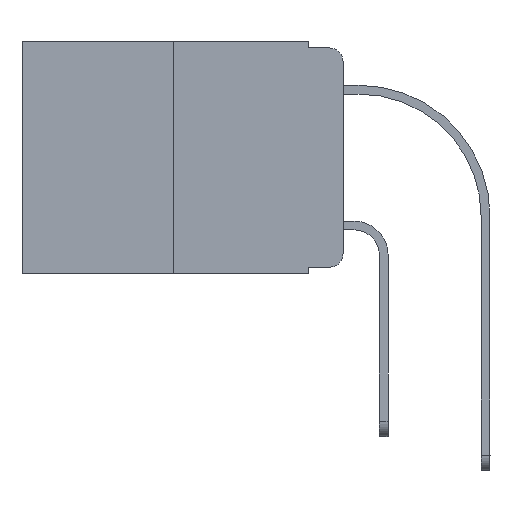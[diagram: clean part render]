
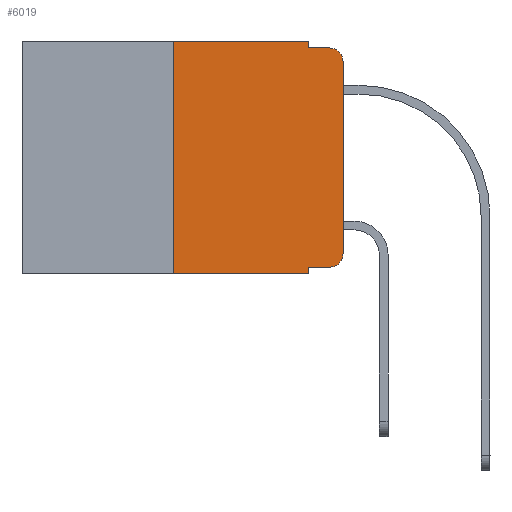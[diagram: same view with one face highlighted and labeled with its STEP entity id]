
A CAD part, left-side view. The second image highlights one B-rep face of the part: STEP entity #6019.
In plain terms, the highlighted planar face has unit normal (-1, 0, 0).
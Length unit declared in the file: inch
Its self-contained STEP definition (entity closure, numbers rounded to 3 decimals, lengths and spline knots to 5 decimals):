
#212 = DIRECTION ( 'NONE',  ( 0., 0., -1. ) ) ;
#283 = EDGE_CURVE ( 'NONE', #6060, #420, #3890, .T. ) ;
#391 = CARTESIAN_POINT ( 'NONE',  ( 0., 0.051, 0. ) ) ;
#420 = VERTEX_POINT ( 'NONE', #11508 ) ;
#975 = ORIENTED_EDGE ( 'NONE', *, *, #1714, .F. ) ;
#992 = VERTEX_POINT ( 'NONE', #1026 ) ;
#1026 = CARTESIAN_POINT ( 'NONE',  ( 0., 0., -0.03 ) ) ;
#1059 = DIRECTION ( 'NONE',  ( 0., -1., 0. ) ) ;
#1162 = AXIS2_PLACEMENT_3D ( 'NONE', #11827, #11709, #3412 ) ;
#1232 = CARTESIAN_POINT ( 'NONE',  ( 0., 0.02, -0.01 ) ) ;
#1286 = EDGE_CURVE ( 'NONE', #6652, #2358, #6255, .T. ) ;
#1702 = EDGE_CURVE ( 'NONE', #2001, #3660, #5364, .T. ) ;
#1714 = EDGE_CURVE ( 'NONE', #7284, #7756, #11695, .T. ) ;
#1765 = ORIENTED_EDGE ( 'NONE', *, *, #10094, .T. ) ;
#1798 = CARTESIAN_POINT ( 'NONE',  ( 0., 0.051, -0.343 ) ) ;
#1846 = LINE ( 'NONE', #4618, #3182 ) ;
#1879 = DIRECTION ( 'NONE',  ( 0., -1., 0. ) ) ;
#1901 = CARTESIAN_POINT ( 'NONE',  ( 0., 0.02, -0.03 ) ) ;
#2001 = VERTEX_POINT ( 'NONE', #391 ) ;
#2096 = FACE_OUTER_BOUND ( 'NONE', #11350, .T. ) ;
#2358 = VERTEX_POINT ( 'NONE', #3750 ) ;
#2893 = DIRECTION ( 'NONE',  ( 0., 0., -1. ) ) ;
#2902 = VECTOR ( 'NONE', #1059, 39.37008 ) ;
#3024 = ORIENTED_EDGE ( 'NONE', *, *, #9170, .F. ) ;
#3182 = VECTOR ( 'NONE', #11875, 39.37008 ) ;
#3412 = DIRECTION ( 'NONE',  ( 0., 0., -1. ) ) ;
#3455 = CARTESIAN_POINT ( 'NONE',  ( 0., 0.473, -0.343 ) ) ;
#3458 = CARTESIAN_POINT ( 'NONE',  ( 0., 0.051, 0. ) ) ;
#3474 = EDGE_CURVE ( 'NONE', #2358, #992, #1846, .T. ) ;
#3660 = VERTEX_POINT ( 'NONE', #6199 ) ;
#3750 = CARTESIAN_POINT ( 'NONE',  ( 0., 0., -0.313 ) ) ;
#3890 = LINE ( 'NONE', #7535, #11661 ) ;
#4532 = CARTESIAN_POINT ( 'NONE',  ( 0., 0.051, -0.333 ) ) ;
#4618 = CARTESIAN_POINT ( 'NONE',  ( 0., 0., 0. ) ) ;
#4701 = EDGE_CURVE ( 'NONE', #420, #2001, #7469, .T. ) ;
#4981 = ORIENTED_EDGE ( 'NONE', *, *, #283, .F. ) ;
#5364 = LINE ( 'NONE', #8975, #10150 ) ;
#5418 = DIRECTION ( 'NONE',  ( 0., -1., 0. ) ) ;
#5606 = VECTOR ( 'NONE', #5418, 39.37008 ) ;
#5631 = CARTESIAN_POINT ( 'NONE',  ( 0., 0.051, -0.333 ) ) ;
#6019 = ADVANCED_FACE ( 'NONE', ( #2096 ), #10368, .F. ) ;
#6060 = VERTEX_POINT ( 'NONE', #7714 ) ;
#6199 = CARTESIAN_POINT ( 'NONE',  ( 0., 0.051, -0.01 ) ) ;
#6204 = ORIENTED_EDGE ( 'NONE', *, *, #1702, .F. ) ;
#6255 = CIRCLE ( 'NONE', #1162, 0.02 ) ;
#6346 = EDGE_CURVE ( 'NONE', #6060, #7756, #7303, .T. ) ;
#6467 = EDGE_CURVE ( 'NONE', #992, #6727, #8547, .T. ) ;
#6652 = VERTEX_POINT ( 'NONE', #8897 ) ;
#6663 = LINE ( 'NONE', #5631, #8895 ) ;
#6727 = VERTEX_POINT ( 'NONE', #1232 ) ;
#7284 = VERTEX_POINT ( 'NONE', #4532 ) ;
#7303 = LINE ( 'NONE', #3455, #5606 ) ;
#7469 = LINE ( 'NONE', #8369, #7937 ) ;
#7481 = DIRECTION ( 'NONE',  ( 0., 0., 1. ) ) ;
#7535 = CARTESIAN_POINT ( 'NONE',  ( 0., 0.25, 0. ) ) ;
#7714 = CARTESIAN_POINT ( 'NONE',  ( 0., 0.25, -0.343 ) ) ;
#7721 = ORIENTED_EDGE ( 'NONE', *, *, #6346, .T. ) ;
#7756 = VERTEX_POINT ( 'NONE', #1798 ) ;
#7937 = VECTOR ( 'NONE', #9825, 39.37008 ) ;
#7967 = AXIS2_PLACEMENT_3D ( 'NONE', #8620, #9459, #212 ) ;
#8020 = DIRECTION ( 'NONE',  ( 0., 0., -1. ) ) ;
#8075 = DIRECTION ( 'NONE',  ( 0., 0., -1. ) ) ;
#8369 = CARTESIAN_POINT ( 'NONE',  ( 0., 0.473, 0. ) ) ;
#8481 = CARTESIAN_POINT ( 'NONE',  ( 0., 0.051, -0.01 ) ) ;
#8547 = CIRCLE ( 'NONE', #9123, 0.02 ) ;
#8620 = CARTESIAN_POINT ( 'NONE',  ( 0., 0.473, 0. ) ) ;
#8895 = VECTOR ( 'NONE', #1879, 39.37008 ) ;
#8897 = CARTESIAN_POINT ( 'NONE',  ( 0., 0.02, -0.333 ) ) ;
#8975 = CARTESIAN_POINT ( 'NONE',  ( 0., 0.051, 0. ) ) ;
#9123 = AXIS2_PLACEMENT_3D ( 'NONE', #1901, #9445, #2893 ) ;
#9170 = EDGE_CURVE ( 'NONE', #3660, #6727, #9513, .T. ) ;
#9445 = DIRECTION ( 'NONE',  ( -1., 0., 0. ) ) ;
#9459 = DIRECTION ( 'NONE',  ( 1., 0., 0. ) ) ;
#9513 = LINE ( 'NONE', #8481, #2902 ) ;
#9541 = ORIENTED_EDGE ( 'NONE', *, *, #3474, .T. ) ;
#9825 = DIRECTION ( 'NONE',  ( 0., -1., 0. ) ) ;
#10094 = EDGE_CURVE ( 'NONE', #7284, #6652, #6663, .T. ) ;
#10150 = VECTOR ( 'NONE', #8020, 39.37008 ) ;
#10368 = PLANE ( 'NONE',  #7967 ) ;
#10678 = ORIENTED_EDGE ( 'NONE', *, *, #1286, .T. ) ;
#10797 = ORIENTED_EDGE ( 'NONE', *, *, #6467, .T. ) ;
#10972 = ORIENTED_EDGE ( 'NONE', *, *, #4701, .F. ) ;
#11350 = EDGE_LOOP ( 'NONE', ( #9541, #10797, #3024, #6204, #10972, #4981, #7721, #975, #1765, #10678 ) ) ;
#11508 = CARTESIAN_POINT ( 'NONE',  ( 0., 0.25, 0. ) ) ;
#11661 = VECTOR ( 'NONE', #7481, 39.37008 ) ;
#11695 = LINE ( 'NONE', #3458, #11892 ) ;
#11709 = DIRECTION ( 'NONE',  ( -1., 0., 0. ) ) ;
#11827 = CARTESIAN_POINT ( 'NONE',  ( 0., 0.02, -0.313 ) ) ;
#11875 = DIRECTION ( 'NONE',  ( 0., 0., 1. ) ) ;
#11892 = VECTOR ( 'NONE', #8075, 39.37008 ) ;
